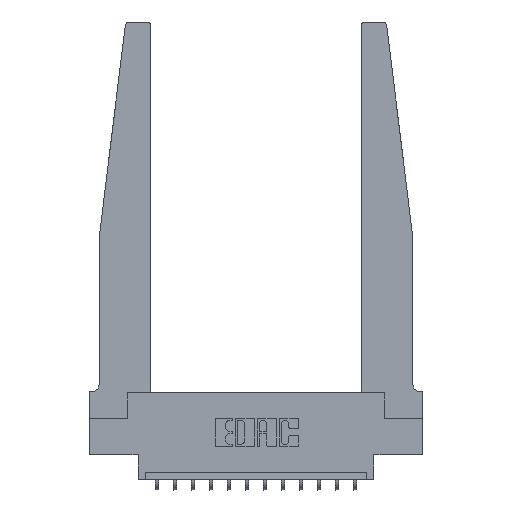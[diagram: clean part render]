
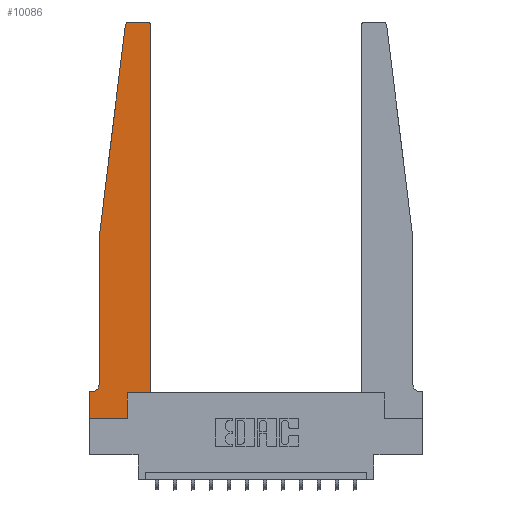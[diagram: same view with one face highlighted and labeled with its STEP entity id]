
A CAD part, top view. The second image highlights one B-rep face of the part: STEP entity #10086.
In plain terms, the highlighted planar face has unit normal (0, 0, 1).
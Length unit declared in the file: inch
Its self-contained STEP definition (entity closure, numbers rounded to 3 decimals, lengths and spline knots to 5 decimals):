
#143 = DIRECTION ( 'NONE',  ( 0., 1., 0. ) ) ;
#364 = EDGE_LOOP ( 'NONE', ( #2166, #1993, #7411, #8778, #12051, #2462, #8973, #3068, #15130, #8032, #14184, #6346 ) ) ;
#463 = VECTOR ( 'NONE', #16067, 39.37008 ) ;
#774 = DIRECTION ( 'NONE',  ( -0.122, -0.992, 0. ) ) ;
#863 = VERTEX_POINT ( 'NONE', #2859 ) ;
#964 = PLANE ( 'NONE',  #7740 ) ;
#1053 = EDGE_CURVE ( 'NONE', #6033, #12426, #2785, .T. ) ;
#1380 = DIRECTION ( 'NONE',  ( 0., 1., 0. ) ) ;
#1736 = DIRECTION ( 'NONE',  ( 1., 0., 0. ) ) ;
#1750 = EDGE_CURVE ( 'NONE', #12426, #6364, #5983, .T. ) ;
#1781 = LINE ( 'NONE', #12124, #14454 ) ;
#1803 = CARTESIAN_POINT ( 'NONE',  ( 0., 0., 0.37 ) ) ;
#1993 = ORIENTED_EDGE ( 'NONE', *, *, #7564, .T. ) ;
#2054 = EDGE_CURVE ( 'NONE', #10772, #15693, #14999, .T. ) ;
#2166 = ORIENTED_EDGE ( 'NONE', *, *, #2054, .T. ) ;
#2462 = ORIENTED_EDGE ( 'NONE', *, *, #10981, .T. ) ;
#2552 = VECTOR ( 'NONE', #13932, 39.37008 ) ;
#2785 = LINE ( 'NONE', #1803, #12043 ) ;
#2859 = CARTESIAN_POINT ( 'NONE',  ( 0.2605, 0.18, 0.37 ) ) ;
#2905 = VECTOR ( 'NONE', #143, 39.37008 ) ;
#2993 = CARTESIAN_POINT ( 'NONE',  ( 0.425, 0.18, 0.37 ) ) ;
#3004 = CIRCLE ( 'NONE', #4293, 0.03 ) ;
#3006 = LINE ( 'NONE', #2993, #8945 ) ;
#3068 = ORIENTED_EDGE ( 'NONE', *, *, #1750, .T. ) ;
#3176 = DIRECTION ( 'NONE',  ( -1., 0., 0. ) ) ;
#3300 = EDGE_CURVE ( 'NONE', #10210, #6373, #12206, .T. ) ;
#3592 = CARTESIAN_POINT ( 'NONE',  ( 0.24675, 2.72367, 0.37 ) ) ;
#3646 = CARTESIAN_POINT ( 'NONE',  ( 0.27653, 2.72, 0.37 ) ) ;
#4293 = AXIS2_PLACEMENT_3D ( 'NONE', #13759, #6253, #15030 ) ;
#4352 = EDGE_CURVE ( 'NONE', #11531, #10210, #10625, .T. ) ;
#4367 = VERTEX_POINT ( 'NONE', #8543 ) ;
#4441 = CARTESIAN_POINT ( 'NONE',  ( 0., 0.1875, 0.37 ) ) ;
#4463 = CIRCLE ( 'NONE', #6045, 0.03 ) ;
#4969 = DIRECTION ( 'NONE',  ( 1., 0., 0. ) ) ;
#5054 = CARTESIAN_POINT ( 'NONE',  ( 0.2605, 0., 0.37 ) ) ;
#5066 = AXIS2_PLACEMENT_3D ( 'NONE', #5738, #14492, #6992 ) ;
#5173 = CARTESIAN_POINT ( 'NONE',  ( 0., 0., 0.37 ) ) ;
#5347 = FACE_OUTER_BOUND ( 'NONE', #364, .T. ) ;
#5738 = CARTESIAN_POINT ( 'NONE',  ( 0.015, 0.2375, 0.37 ) ) ;
#5983 = LINE ( 'NONE', #5173, #2552 ) ;
#6033 = VERTEX_POINT ( 'NONE', #4441 ) ;
#6045 = AXIS2_PLACEMENT_3D ( 'NONE', #3646, #12430, #4969 ) ;
#6104 = VECTOR ( 'NONE', #10666, 39.37008 ) ;
#6164 = DIRECTION ( 'NONE',  ( 1., 0., 0. ) ) ;
#6248 = CARTESIAN_POINT ( 'NONE',  ( 0.425, 0.18, 0.37 ) ) ;
#6253 = DIRECTION ( 'NONE',  ( 0., 0., 1. ) ) ;
#6337 = VERTEX_POINT ( 'NONE', #6248 ) ;
#6346 = ORIENTED_EDGE ( 'NONE', *, *, #13743, .T. ) ;
#6362 = CARTESIAN_POINT ( 'NONE',  ( 0.015, 0.1875, 0.37 ) ) ;
#6364 = VERTEX_POINT ( 'NONE', #5054 ) ;
#6373 = VERTEX_POINT ( 'NONE', #6362 ) ;
#6576 = CARTESIAN_POINT ( 'NONE',  ( 0.425, 0.18, 0.37 ) ) ;
#6992 = DIRECTION ( 'NONE',  ( -1., 0., 0. ) ) ;
#7120 = VECTOR ( 'NONE', #1380, 39.37008 ) ;
#7411 = ORIENTED_EDGE ( 'NONE', *, *, #8533, .T. ) ;
#7564 = EDGE_CURVE ( 'NONE', #15693, #16120, #4463, .T. ) ;
#7740 = AXIS2_PLACEMENT_3D ( 'NONE', #13605, #13655, #6164 ) ;
#8032 = ORIENTED_EDGE ( 'NONE', *, *, #14594, .T. ) ;
#8318 = VECTOR ( 'NONE', #3176, 39.37008 ) ;
#8533 = EDGE_CURVE ( 'NONE', #16120, #11531, #1781, .T. ) ;
#8543 = CARTESIAN_POINT ( 'NONE',  ( 0.425, 2.72, 0.37 ) ) ;
#8778 = ORIENTED_EDGE ( 'NONE', *, *, #4352, .T. ) ;
#8945 = VECTOR ( 'NONE', #1736, 39.37008 ) ;
#8973 = ORIENTED_EDGE ( 'NONE', *, *, #1053, .T. ) ;
#9299 = CARTESIAN_POINT ( 'NONE',  ( 0.065, 1.25, 0.37 ) ) ;
#9386 = DIRECTION ( 'NONE',  ( 0., -1., 0. ) ) ;
#9422 = CARTESIAN_POINT ( 'NONE',  ( 0.065, 0.1875, 0.37 ) ) ;
#9442 = CARTESIAN_POINT ( 'NONE',  ( 0.25, 2.75, 0.37 ) ) ;
#9659 = EDGE_CURVE ( 'NONE', #6364, #863, #10445, .T. ) ;
#9813 = CARTESIAN_POINT ( 'NONE',  ( 0., 0., 0.37 ) ) ;
#10086 = ADVANCED_FACE ( 'NONE', ( #5347 ), #964, .T. ) ;
#10210 = VERTEX_POINT ( 'NONE', #15153 ) ;
#10445 = LINE ( 'NONE', #14005, #7120 ) ;
#10625 = LINE ( 'NONE', #14810, #463 ) ;
#10666 = DIRECTION ( 'NONE',  ( -1., 0., 0. ) ) ;
#10772 = VERTEX_POINT ( 'NONE', #14086 ) ;
#10788 = EDGE_CURVE ( 'NONE', #6337, #4367, #15927, .T. ) ;
#10981 = EDGE_CURVE ( 'NONE', #6373, #6033, #12744, .T. ) ;
#11531 = VERTEX_POINT ( 'NONE', #9299 ) ;
#12043 = VECTOR ( 'NONE', #9386, 39.37008 ) ;
#12051 = ORIENTED_EDGE ( 'NONE', *, *, #3300, .T. ) ;
#12124 = CARTESIAN_POINT ( 'NONE',  ( 0.065, 1.25, 0.37 ) ) ;
#12206 = CIRCLE ( 'NONE', #5066, 0.05 ) ;
#12426 = VERTEX_POINT ( 'NONE', #9813 ) ;
#12430 = DIRECTION ( 'NONE',  ( 0., 0., 1. ) ) ;
#12673 = CARTESIAN_POINT ( 'NONE',  ( 0.27653, 2.75, 0.37 ) ) ;
#12744 = LINE ( 'NONE', #9422, #6104 ) ;
#13605 = CARTESIAN_POINT ( 'NONE',  ( 0., 0.1875, 0.37 ) ) ;
#13655 = DIRECTION ( 'NONE',  ( 0., 0., 1. ) ) ;
#13743 = EDGE_CURVE ( 'NONE', #4367, #10772, #3004, .T. ) ;
#13759 = CARTESIAN_POINT ( 'NONE',  ( 0.395, 2.72, 0.37 ) ) ;
#13932 = DIRECTION ( 'NONE',  ( 1., 0., 0. ) ) ;
#14005 = CARTESIAN_POINT ( 'NONE',  ( 0.2605, 0.18, 0.37 ) ) ;
#14086 = CARTESIAN_POINT ( 'NONE',  ( 0.395, 2.75, 0.37 ) ) ;
#14184 = ORIENTED_EDGE ( 'NONE', *, *, #10788, .T. ) ;
#14454 = VECTOR ( 'NONE', #774, 39.37008 ) ;
#14492 = DIRECTION ( 'NONE',  ( 0., 0., -1. ) ) ;
#14594 = EDGE_CURVE ( 'NONE', #863, #6337, #3006, .T. ) ;
#14810 = CARTESIAN_POINT ( 'NONE',  ( 0.065, 1.25, 0.37 ) ) ;
#14999 = LINE ( 'NONE', #9442, #8318 ) ;
#15030 = DIRECTION ( 'NONE',  ( 1., 0., 0. ) ) ;
#15130 = ORIENTED_EDGE ( 'NONE', *, *, #9659, .T. ) ;
#15153 = CARTESIAN_POINT ( 'NONE',  ( 0.065, 0.2375, 0.37 ) ) ;
#15693 = VERTEX_POINT ( 'NONE', #12673 ) ;
#15927 = LINE ( 'NONE', #6576, #2905 ) ;
#16067 = DIRECTION ( 'NONE',  ( 0., -1., 0. ) ) ;
#16120 = VERTEX_POINT ( 'NONE', #3592 ) ;
